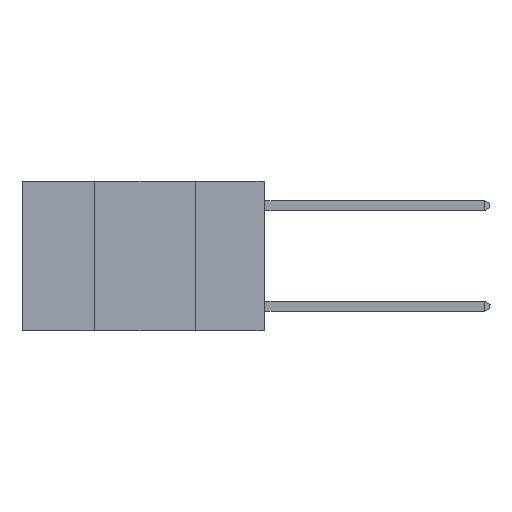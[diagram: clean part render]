
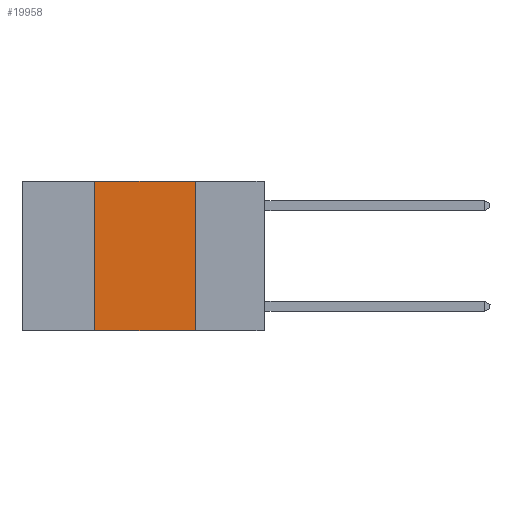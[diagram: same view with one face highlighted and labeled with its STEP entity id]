
A CAD part, left-side view. The second image highlights one B-rep face of the part: STEP entity #19958.
In plain terms, the highlighted planar face has unit normal (-1, 0, 0).
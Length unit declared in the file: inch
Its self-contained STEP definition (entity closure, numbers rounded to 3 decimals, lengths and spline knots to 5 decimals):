
#656 = ORIENTED_EDGE ( 'NONE', *, *, #17841, .F. ) ;
#1319 = DIRECTION ( 'NONE',  ( 0., -1., 0. ) ) ;
#1466 = EDGE_CURVE ( 'NONE', #10654, #18809, #10048, .T. ) ;
#1592 = VERTEX_POINT ( 'NONE', #13356 ) ;
#1614 = FACE_OUTER_BOUND ( 'NONE', #21296, .T. ) ;
#1658 = EDGE_CURVE ( 'NONE', #18809, #20094, #10351, .T. ) ;
#2977 = DIRECTION ( 'NONE',  ( 1., 0., 0. ) ) ;
#3535 = LINE ( 'NONE', #20954, #24203 ) ;
#4747 = VECTOR ( 'NONE', #1319, 39.37008 ) ;
#4816 = ORIENTED_EDGE ( 'NONE', *, *, #1466, .F. ) ;
#4950 = CARTESIAN_POINT ( 'NONE',  ( 0., 0.6, 0. ) ) ;
#5528 = AXIS2_PLACEMENT_3D ( 'NONE', #4950, #2977, #17018 ) ;
#10048 = LINE ( 'NONE', #25485, #4747 ) ;
#10351 = LINE ( 'NONE', #14708, #20398 ) ;
#10654 = VERTEX_POINT ( 'NONE', #21675 ) ;
#11147 = EDGE_CURVE ( 'NONE', #1592, #20094, #3535, .T. ) ;
#13356 = CARTESIAN_POINT ( 'NONE',  ( 0., 0.42, -0.37 ) ) ;
#13733 = VECTOR ( 'NONE', #20048, 39.37008 ) ;
#14329 = LINE ( 'NONE', #25954, #13733 ) ;
#14708 = CARTESIAN_POINT ( 'NONE',  ( 0., 0.17, 0. ) ) ;
#15378 = CARTESIAN_POINT ( 'NONE',  ( 0., 0.17, -0.37 ) ) ;
#17018 = DIRECTION ( 'NONE',  ( 0., 0., -1. ) ) ;
#17806 = DIRECTION ( 'NONE',  ( 0., 0., -1. ) ) ;
#17841 = EDGE_CURVE ( 'NONE', #1592, #10654, #14329, .T. ) ;
#18809 = VERTEX_POINT ( 'NONE', #25630 ) ;
#19036 = DIRECTION ( 'NONE',  ( 0., -1., 0. ) ) ;
#19958 = ADVANCED_FACE ( 'NONE', ( #1614 ), #24880, .F. ) ;
#20048 = DIRECTION ( 'NONE',  ( 0., 0., 1. ) ) ;
#20094 = VERTEX_POINT ( 'NONE', #15378 ) ;
#20398 = VECTOR ( 'NONE', #17806, 39.37008 ) ;
#20954 = CARTESIAN_POINT ( 'NONE',  ( 0., 0.6, -0.37 ) ) ;
#21296 = EDGE_LOOP ( 'NONE', ( #22313, #4816, #656, #24209 ) ) ;
#21675 = CARTESIAN_POINT ( 'NONE',  ( 0., 0.42, 0. ) ) ;
#22313 = ORIENTED_EDGE ( 'NONE', *, *, #1658, .F. ) ;
#24203 = VECTOR ( 'NONE', #19036, 39.37008 ) ;
#24209 = ORIENTED_EDGE ( 'NONE', *, *, #11147, .T. ) ;
#24880 = PLANE ( 'NONE',  #5528 ) ;
#25485 = CARTESIAN_POINT ( 'NONE',  ( 0., 0.6, 0. ) ) ;
#25630 = CARTESIAN_POINT ( 'NONE',  ( 0., 0.17, 0. ) ) ;
#25954 = CARTESIAN_POINT ( 'NONE',  ( 0., 0.42, 0. ) ) ;
